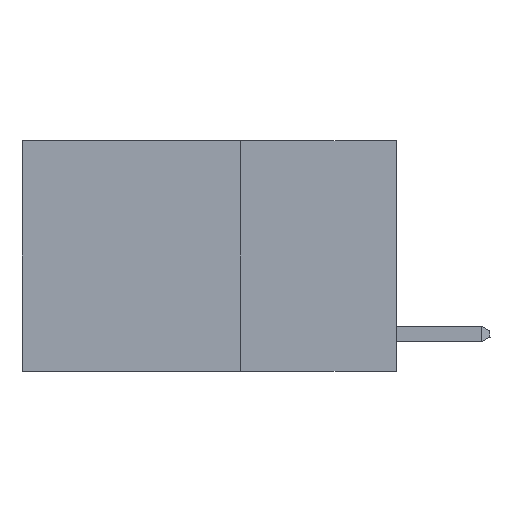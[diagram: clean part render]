
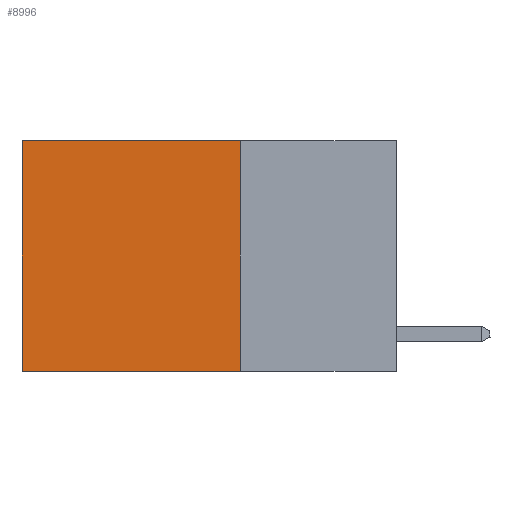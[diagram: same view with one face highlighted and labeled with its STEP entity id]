
A CAD part, left-side view. The second image highlights one B-rep face of the part: STEP entity #8996.
In plain terms, the highlighted planar face has unit normal (-1, 0, 0).
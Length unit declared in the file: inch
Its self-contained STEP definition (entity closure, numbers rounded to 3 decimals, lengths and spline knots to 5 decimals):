
#14 = CARTESIAN_POINT ( 'NONE',  ( 0.2625, 0.25, 0. ) ) ;
#53 = CARTESIAN_POINT ( 'NONE',  ( 0.2625, 0.6, 0. ) ) ;
#316 = ORIENTED_EDGE ( 'NONE', *, *, #10976, .T. ) ;
#370 = ORIENTED_EDGE ( 'NONE', *, *, #2208, .F. ) ;
#514 = FACE_OUTER_BOUND ( 'NONE', #4030, .T. ) ;
#925 = DIRECTION ( 'NONE',  ( 0., 1., 0. ) ) ;
#970 = CARTESIAN_POINT ( 'NONE',  ( 0.2625, 0.25, -0.37 ) ) ;
#1021 = DIRECTION ( 'NONE',  ( 0., 0., -1. ) ) ;
#1166 = CARTESIAN_POINT ( 'NONE',  ( 0.2625, 0.25, 0. ) ) ;
#1231 = CARTESIAN_POINT ( 'NONE',  ( 0.2625, 0.6, -0.37 ) ) ;
#1566 = ORIENTED_EDGE ( 'NONE', *, *, #4531, .F. ) ;
#2045 = CARTESIAN_POINT ( 'NONE',  ( 0.2625, 0.25, 0. ) ) ;
#2208 = EDGE_CURVE ( 'NONE', #10949, #7230, #10143, .T. ) ;
#2834 = VECTOR ( 'NONE', #925, 39.37008 ) ;
#3313 = VERTEX_POINT ( 'NONE', #1231 ) ;
#3608 = AXIS2_PLACEMENT_3D ( 'NONE', #14, #6929, #1021 ) ;
#3907 = ORIENTED_EDGE ( 'NONE', *, *, #10347, .T. ) ;
#4030 = EDGE_LOOP ( 'NONE', ( #316, #1566, #370, #3907 ) ) ;
#4531 = EDGE_CURVE ( 'NONE', #7230, #3313, #7419, .T. ) ;
#4592 = CARTESIAN_POINT ( 'NONE',  ( 0.2625, 0.6, 0. ) ) ;
#5222 = CARTESIAN_POINT ( 'NONE',  ( 0.2625, 0.25, 0. ) ) ;
#5935 = PLANE ( 'NONE',  #3608 ) ;
#5969 = DIRECTION ( 'NONE',  ( 0., 0., -1. ) ) ;
#6929 = DIRECTION ( 'NONE',  ( 1., 0., 0. ) ) ;
#7230 = VERTEX_POINT ( 'NONE', #9839 ) ;
#7247 = LINE ( 'NONE', #53, #11922 ) ;
#7419 = LINE ( 'NONE', #970, #2834 ) ;
#7602 = VECTOR ( 'NONE', #8125, 39.37008 ) ;
#8125 = DIRECTION ( 'NONE',  ( 0., 0., -1. ) ) ;
#8996 = ADVANCED_FACE ( 'NONE', ( #514 ), #5935, .F. ) ;
#9008 = DIRECTION ( 'NONE',  ( 0., 1., 0. ) ) ;
#9357 = LINE ( 'NONE', #1166, #9657 ) ;
#9657 = VECTOR ( 'NONE', #9008, 39.37008 ) ;
#9839 = CARTESIAN_POINT ( 'NONE',  ( 0.2625, 0.25, -0.37 ) ) ;
#10006 = VERTEX_POINT ( 'NONE', #4592 ) ;
#10143 = LINE ( 'NONE', #5222, #7602 ) ;
#10347 = EDGE_CURVE ( 'NONE', #10949, #10006, #9357, .T. ) ;
#10949 = VERTEX_POINT ( 'NONE', #2045 ) ;
#10976 = EDGE_CURVE ( 'NONE', #10006, #3313, #7247, .T. ) ;
#11922 = VECTOR ( 'NONE', #5969, 39.37008 ) ;
